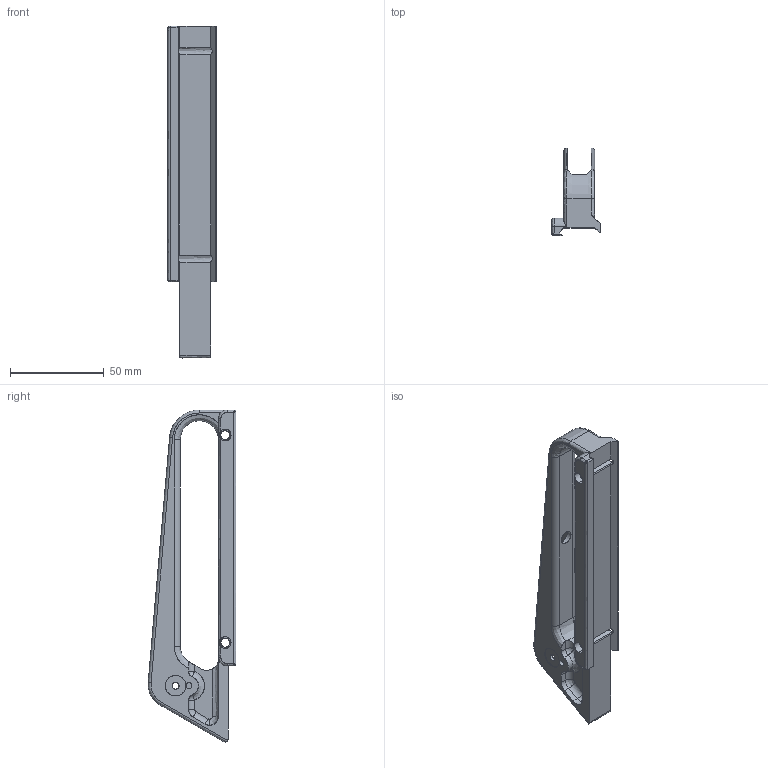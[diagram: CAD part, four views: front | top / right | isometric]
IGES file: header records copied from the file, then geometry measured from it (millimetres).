
Start section: SolidWorks IGES FILE using analytic representation for surfaces
Global section: file name: A1_De_Handle.IGS; native system: SolidWorks 2004 by SolidWorks Corporation; preprocessor: Version 5.3; author: Me; date: 040220.211616; units: inch
Bounding box: 25.65 x 46.73 x 176.64 mm (x, y, z)
Surface area: 25097.7 mm2 (no closed solid volume)
Topology: 0 solids, 0 shells, 145 faces, 2100 edges, 2098 vertices
Faces by surface type: revolution 75, bspline 70
